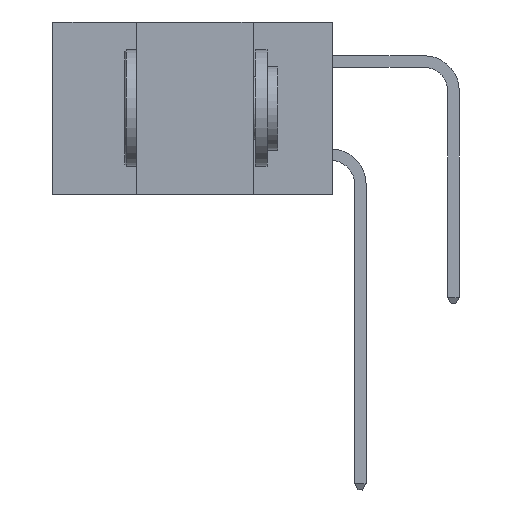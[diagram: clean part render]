
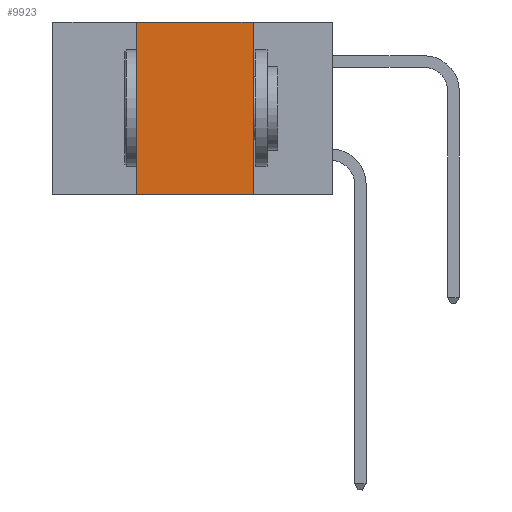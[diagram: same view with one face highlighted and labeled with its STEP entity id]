
A CAD part, left-side view. The second image highlights one B-rep face of the part: STEP entity #9923.
In plain terms, the highlighted planar face has unit normal (-1, 0, 0).
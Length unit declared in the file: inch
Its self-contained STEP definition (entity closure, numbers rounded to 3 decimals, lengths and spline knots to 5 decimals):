
#27 = ORIENTED_EDGE ( 'NONE', *, *, #5468, .T. ) ;
#1389 = CARTESIAN_POINT ( 'NONE',  ( 0., 0.6, -0.37 ) ) ;
#2075 = ORIENTED_EDGE ( 'NONE', *, *, #9776, .F. ) ;
#2172 = ORIENTED_EDGE ( 'NONE', *, *, #14289, .F. ) ;
#2483 = DIRECTION ( 'NONE',  ( 0., 0., -1. ) ) ;
#2956 = ORIENTED_EDGE ( 'NONE', *, *, #14364, .F. ) ;
#3455 = DIRECTION ( 'NONE',  ( 0., 0., 1. ) ) ;
#4136 = DIRECTION ( 'NONE',  ( 0., 0., -1. ) ) ;
#4430 = VECTOR ( 'NONE', #4136, 39.37008 ) ;
#4437 = PLANE ( 'NONE',  #6250 ) ;
#5291 = VERTEX_POINT ( 'NONE', #5433 ) ;
#5433 = CARTESIAN_POINT ( 'NONE',  ( 0., 0.17, -0.37 ) ) ;
#5468 = EDGE_CURVE ( 'NONE', #7775, #5291, #6853, .T. ) ;
#5689 = FACE_OUTER_BOUND ( 'NONE', #13506, .T. ) ;
#5860 = DIRECTION ( 'NONE',  ( 0., -1., 0. ) ) ;
#5948 = LINE ( 'NONE', #13122, #10366 ) ;
#6250 = AXIS2_PLACEMENT_3D ( 'NONE', #10224, #13930, #2483 ) ;
#6853 = LINE ( 'NONE', #1389, #8697 ) ;
#7341 = CARTESIAN_POINT ( 'NONE',  ( 0., 0.42, 0. ) ) ;
#7775 = VERTEX_POINT ( 'NONE', #13130 ) ;
#8183 = DIRECTION ( 'NONE',  ( 0., -1., 0. ) ) ;
#8363 = VERTEX_POINT ( 'NONE', #7341 ) ;
#8668 = CARTESIAN_POINT ( 'NONE',  ( 0., 0.17, -0.37 ) ) ;
#8697 = VECTOR ( 'NONE', #5860, 39.37008 ) ;
#9776 = EDGE_CURVE ( 'NONE', #7775, #8363, #14090, .T. ) ;
#9923 = ADVANCED_FACE ( 'NONE', ( #5689 ), #4437, .F. ) ;
#10224 = CARTESIAN_POINT ( 'NONE',  ( 0., 0.6, 0. ) ) ;
#10366 = VECTOR ( 'NONE', #8183, 39.37008 ) ;
#10490 = LINE ( 'NONE', #8668, #4430 ) ;
#10756 = CARTESIAN_POINT ( 'NONE',  ( 0., 0.42, -0.37 ) ) ;
#10773 = VECTOR ( 'NONE', #3455, 39.37008 ) ;
#11306 = VERTEX_POINT ( 'NONE', #13437 ) ;
#13122 = CARTESIAN_POINT ( 'NONE',  ( 0., 0.6, 0. ) ) ;
#13130 = CARTESIAN_POINT ( 'NONE',  ( 0., 0.42, -0.37 ) ) ;
#13437 = CARTESIAN_POINT ( 'NONE',  ( 0., 0.17, 0. ) ) ;
#13506 = EDGE_LOOP ( 'NONE', ( #2172, #2956, #2075, #27 ) ) ;
#13930 = DIRECTION ( 'NONE',  ( 1., 0., 0. ) ) ;
#14090 = LINE ( 'NONE', #10756, #10773 ) ;
#14289 = EDGE_CURVE ( 'NONE', #11306, #5291, #10490, .T. ) ;
#14364 = EDGE_CURVE ( 'NONE', #8363, #11306, #5948, .T. ) ;
